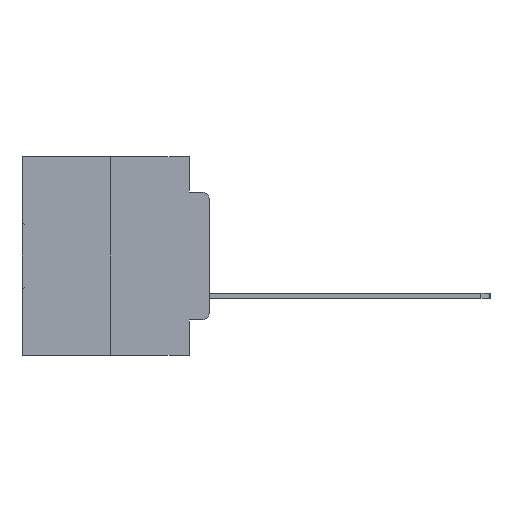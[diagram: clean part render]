
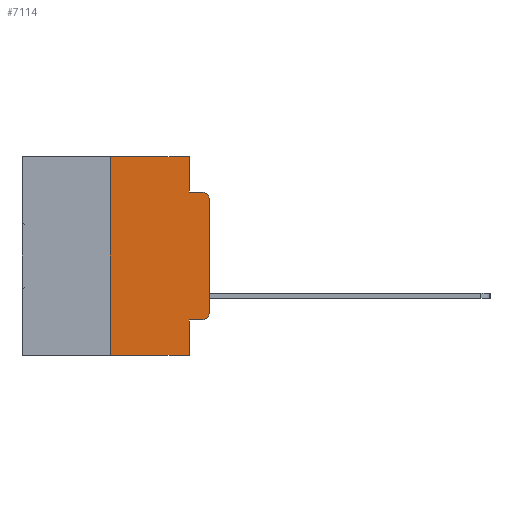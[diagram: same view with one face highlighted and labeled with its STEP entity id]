
A CAD part, left-side view. The second image highlights one B-rep face of the part: STEP entity #7114.
In plain terms, the highlighted planar face has unit normal (-1, 0, 0).
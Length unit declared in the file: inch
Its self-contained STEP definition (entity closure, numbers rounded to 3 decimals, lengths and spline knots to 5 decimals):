
#265 = EDGE_CURVE ( 'NONE', #5319, #18083, #15991, .T. ) ;
#605 = EDGE_CURVE ( 'NONE', #22632, #26590, #5904, .T. ) ;
#1774 = DIRECTION ( 'NONE',  ( 1., 0., 0. ) ) ;
#1779 = DIRECTION ( 'NONE',  ( 0., 0., -1. ) ) ;
#2438 = DIRECTION ( 'NONE',  ( 0., 0., 1. ) ) ;
#2523 = LINE ( 'NONE', #24528, #27938 ) ;
#3696 = DIRECTION ( 'NONE',  ( 0., -1., 0. ) ) ;
#3768 = CARTESIAN_POINT ( 'NONE',  ( 0., 0.25, -0.5 ) ) ;
#3796 = FACE_OUTER_BOUND ( 'NONE', #21710, .T. ) ;
#3909 = CARTESIAN_POINT ( 'NONE',  ( 0., 0.473, 0. ) ) ;
#3946 = CARTESIAN_POINT ( 'NONE',  ( 0., 0.25, 0. ) ) ;
#4045 = AXIS2_PLACEMENT_3D ( 'NONE', #30765, #16214, #1779 ) ;
#4358 = VERTEX_POINT ( 'NONE', #18877 ) ;
#4455 = ORIENTED_EDGE ( 'NONE', *, *, #19312, .F. ) ;
#4485 = CARTESIAN_POINT ( 'NONE',  ( 0., 0.02, -0.4115 ) ) ;
#4609 = EDGE_CURVE ( 'NONE', #26590, #24826, #31192, .T. ) ;
#4869 = EDGE_CURVE ( 'NONE', #5482, #24891, #24374, .T. ) ;
#4945 = EDGE_CURVE ( 'NONE', #9303, #5319, #15590, .T. ) ;
#5213 = ORIENTED_EDGE ( 'NONE', *, *, #19777, .F. ) ;
#5319 = VERTEX_POINT ( 'NONE', #17880 ) ;
#5448 = CARTESIAN_POINT ( 'NONE',  ( 0., 0., -0.1085 ) ) ;
#5482 = VERTEX_POINT ( 'NONE', #3768 ) ;
#5904 = LINE ( 'NONE', #8423, #24757 ) ;
#6106 = VERTEX_POINT ( 'NONE', #5448 ) ;
#6483 = DIRECTION ( 'NONE',  ( 0., 0., -1. ) ) ;
#6542 = LINE ( 'NONE', #7959, #18896 ) ;
#7114 = ADVANCED_FACE ( 'NONE', ( #3796 ), #28794, .F. ) ;
#7395 = ORIENTED_EDGE ( 'NONE', *, *, #605, .T. ) ;
#7456 = CIRCLE ( 'NONE', #4045, 0.02 ) ;
#7556 = CARTESIAN_POINT ( 'NONE',  ( 0., 0.02, -0.3915 ) ) ;
#7959 = CARTESIAN_POINT ( 'NONE',  ( 0., 0.051, -0.0885 ) ) ;
#8180 = DIRECTION ( 'NONE',  ( 0., -1., 0. ) ) ;
#8423 = CARTESIAN_POINT ( 'NONE',  ( 0., 0.051, -0.4115 ) ) ;
#9030 = VECTOR ( 'NONE', #23508, 39.37008 ) ;
#9303 = VERTEX_POINT ( 'NONE', #3946 ) ;
#9559 = LINE ( 'NONE', #21228, #16108 ) ;
#9967 = ORIENTED_EDGE ( 'NONE', *, *, #31666, .T. ) ;
#10041 = DIRECTION ( 'NONE',  ( 0., 0., -1. ) ) ;
#10082 = CARTESIAN_POINT ( 'NONE',  ( 0., 0.051, -0.4115 ) ) ;
#10578 = EDGE_CURVE ( 'NONE', #22632, #24891, #9559, .T. ) ;
#10596 = VECTOR ( 'NONE', #3696, 39.37008 ) ;
#10797 = LINE ( 'NONE', #29549, #16576 ) ;
#10816 = EDGE_CURVE ( 'NONE', #24826, #6106, #2523, .T. ) ;
#13419 = ORIENTED_EDGE ( 'NONE', *, *, #10578, .F. ) ;
#14936 = CARTESIAN_POINT ( 'NONE',  ( 0., 0.051, 0. ) ) ;
#14943 = DIRECTION ( 'NONE',  ( 0., 0., 1. ) ) ;
#14980 = DIRECTION ( 'NONE',  ( 0., 0., -1. ) ) ;
#15230 = VECTOR ( 'NONE', #14980, 39.37008 ) ;
#15590 = LINE ( 'NONE', #3909, #9030 ) ;
#15991 = LINE ( 'NONE', #14936, #15230 ) ;
#16108 = VECTOR ( 'NONE', #6483, 39.37008 ) ;
#16214 = DIRECTION ( 'NONE',  ( -1., 0., 0. ) ) ;
#16576 = VECTOR ( 'NONE', #14943, 39.37008 ) ;
#16948 = ORIENTED_EDGE ( 'NONE', *, *, #4869, .T. ) ;
#17880 = CARTESIAN_POINT ( 'NONE',  ( 0., 0.051, 0. ) ) ;
#17942 = AXIS2_PLACEMENT_3D ( 'NONE', #7556, #24716, #10041 ) ;
#18083 = VERTEX_POINT ( 'NONE', #19957 ) ;
#18877 = CARTESIAN_POINT ( 'NONE',  ( 0., 0.02, -0.0885 ) ) ;
#18896 = VECTOR ( 'NONE', #8180, 39.37008 ) ;
#19107 = DIRECTION ( 'NONE',  ( 0., 0., -1. ) ) ;
#19312 = EDGE_CURVE ( 'NONE', #18083, #4358, #6542, .T. ) ;
#19777 = EDGE_CURVE ( 'NONE', #5482, #9303, #10797, .T. ) ;
#19957 = CARTESIAN_POINT ( 'NONE',  ( 0., 0.051, -0.0885 ) ) ;
#20040 = ORIENTED_EDGE ( 'NONE', *, *, #265, .F. ) ;
#20204 = ORIENTED_EDGE ( 'NONE', *, *, #4609, .T. ) ;
#21228 = CARTESIAN_POINT ( 'NONE',  ( 0., 0.051, 0. ) ) ;
#21710 = EDGE_LOOP ( 'NONE', ( #29865, #9967, #4455, #20040, #22453, #5213, #16948, #13419, #7395, #20204 ) ) ;
#22453 = ORIENTED_EDGE ( 'NONE', *, *, #4945, .F. ) ;
#22632 = VERTEX_POINT ( 'NONE', #10082 ) ;
#23508 = DIRECTION ( 'NONE',  ( 0., -1., 0. ) ) ;
#24374 = LINE ( 'NONE', #30610, #10596 ) ;
#24528 = CARTESIAN_POINT ( 'NONE',  ( 0., 0., 0. ) ) ;
#24716 = DIRECTION ( 'NONE',  ( -1., 0., 0. ) ) ;
#24757 = VECTOR ( 'NONE', #26391, 39.37008 ) ;
#24826 = VERTEX_POINT ( 'NONE', #26614 ) ;
#24891 = VERTEX_POINT ( 'NONE', #29366 ) ;
#26391 = DIRECTION ( 'NONE',  ( 0., -1., 0. ) ) ;
#26590 = VERTEX_POINT ( 'NONE', #4485 ) ;
#26614 = CARTESIAN_POINT ( 'NONE',  ( 0., 0., -0.3915 ) ) ;
#27774 = AXIS2_PLACEMENT_3D ( 'NONE', #31183, #1774, #19107 ) ;
#27938 = VECTOR ( 'NONE', #2438, 39.37008 ) ;
#28794 = PLANE ( 'NONE',  #27774 ) ;
#29366 = CARTESIAN_POINT ( 'NONE',  ( 0., 0.051, -0.5 ) ) ;
#29549 = CARTESIAN_POINT ( 'NONE',  ( 0., 0.25, 0. ) ) ;
#29865 = ORIENTED_EDGE ( 'NONE', *, *, #10816, .T. ) ;
#30610 = CARTESIAN_POINT ( 'NONE',  ( 0., 0.473, -0.5 ) ) ;
#30765 = CARTESIAN_POINT ( 'NONE',  ( 0., 0.02, -0.1085 ) ) ;
#31183 = CARTESIAN_POINT ( 'NONE',  ( 0., 0.473, 0. ) ) ;
#31192 = CIRCLE ( 'NONE', #17942, 0.02 ) ;
#31666 = EDGE_CURVE ( 'NONE', #6106, #4358, #7456, .T. ) ;
